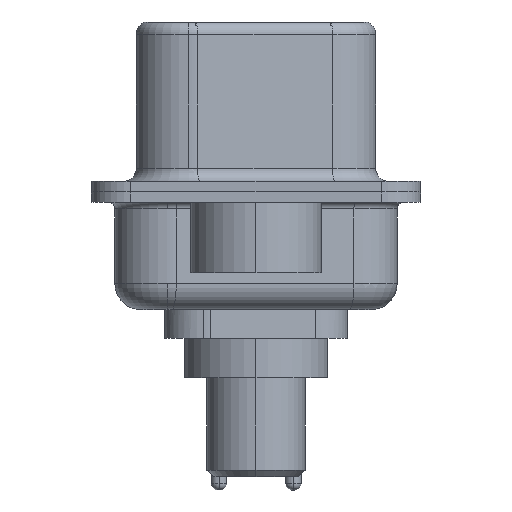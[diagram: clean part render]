
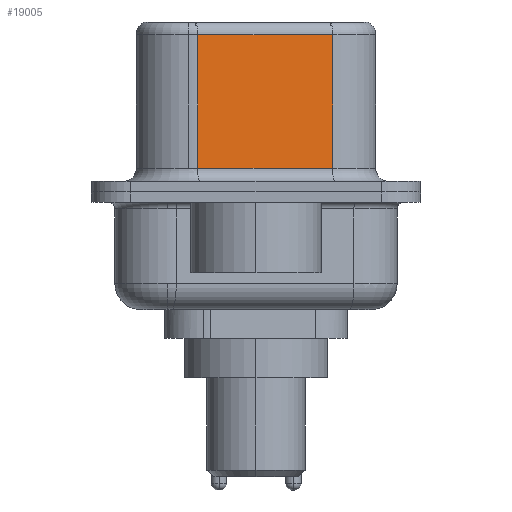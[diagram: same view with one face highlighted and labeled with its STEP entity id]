
A CAD part, left-side view. The second image highlights one B-rep face of the part: STEP entity #19005.
In plain terms, the highlighted planar face has unit normal (-0.985, -0.174, 0).
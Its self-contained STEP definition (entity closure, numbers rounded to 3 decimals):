
#2293 = ORIENTED_EDGE ( 'NONE', *, *, #4204, .T. ) ;
#2730 = CARTESIAN_POINT ( 'NONE',  ( 4.58, -2.927, 0.9 ) ) ;
#2772 = EDGE_CURVE ( 'NONE', #11079, #14261, #15086, .T. ) ;
#3467 = DIRECTION ( 'NONE',  ( 0.985, 0.174, 0. ) ) ;
#4020 = CARTESIAN_POINT ( 'NONE',  ( 3.67, 2.233, 0.9 ) ) ;
#4082 = ORIENTED_EDGE ( 'NONE', *, *, #2772, .F. ) ;
#4204 = EDGE_CURVE ( 'NONE', #15297, #4407, #15969, .T. ) ;
#4341 = VECTOR ( 'NONE', #16740, 1000. ) ;
#4407 = VERTEX_POINT ( 'NONE', #4020 ) ;
#4731 = CARTESIAN_POINT ( 'NONE',  ( 4.58, -2.927, 0.9 ) ) ;
#6775 = DIRECTION ( 'NONE',  ( 0., 0., -1. ) ) ;
#8323 = ORIENTED_EDGE ( 'NONE', *, *, #20519, .T. ) ;
#8764 = CARTESIAN_POINT ( 'NONE',  ( 3.67, 2.233, 6.52 ) ) ;
#9655 = LINE ( 'NONE', #4731, #4341 ) ;
#11079 = VERTEX_POINT ( 'NONE', #22151 ) ;
#14261 = VERTEX_POINT ( 'NONE', #2730 ) ;
#15086 = LINE ( 'NONE', #15538, #25101 ) ;
#15122 = ORIENTED_EDGE ( 'NONE', *, *, #18763, .T. ) ;
#15297 = VERTEX_POINT ( 'NONE', #23838 ) ;
#15476 = CARTESIAN_POINT ( 'NONE',  ( 4.58, -2.927, 6.52 ) ) ;
#15538 = CARTESIAN_POINT ( 'NONE',  ( 4.58, -2.927, 6.52 ) ) ;
#15798 = EDGE_LOOP ( 'NONE', ( #4082, #8323, #2293, #15122 ) ) ;
#15969 = LINE ( 'NONE', #8764, #25988 ) ;
#16740 = DIRECTION ( 'NONE',  ( 0.174, -0.985, 0. ) ) ;
#16948 = AXIS2_PLACEMENT_3D ( 'NONE', #15476, #3467, #17519 ) ;
#17519 = DIRECTION ( 'NONE',  ( -0.174, 0.985, 0. ) ) ;
#17963 = DIRECTION ( 'NONE',  ( 0., 0., -1. ) ) ;
#18747 = LINE ( 'NONE', #22234, #22768 ) ;
#18763 = EDGE_CURVE ( 'NONE', #4407, #14261, #9655, .T. ) ;
#19005 = ADVANCED_FACE ( 'NONE', ( #25309 ), #23455, .F. ) ;
#20519 = EDGE_CURVE ( 'NONE', #11079, #15297, #18747, .T. ) ;
#22151 = CARTESIAN_POINT ( 'NONE',  ( 4.58, -2.927, 6.02 ) ) ;
#22234 = CARTESIAN_POINT ( 'NONE',  ( 4.58, -2.927, 6.02 ) ) ;
#22768 = VECTOR ( 'NONE', #24257, 1000. ) ;
#23455 = PLANE ( 'NONE',  #16948 ) ;
#23838 = CARTESIAN_POINT ( 'NONE',  ( 3.67, 2.233, 6.02 ) ) ;
#24257 = DIRECTION ( 'NONE',  ( -0.174, 0.985, 0. ) ) ;
#25101 = VECTOR ( 'NONE', #17963, 1000. ) ;
#25309 = FACE_OUTER_BOUND ( 'NONE', #15798, .T. ) ;
#25988 = VECTOR ( 'NONE', #6775, 1000. ) ;
